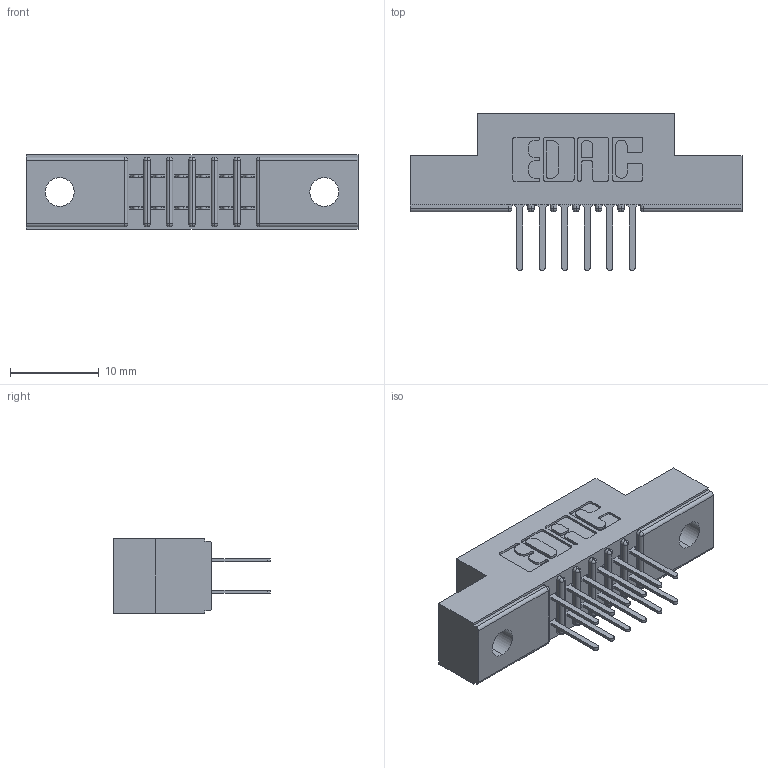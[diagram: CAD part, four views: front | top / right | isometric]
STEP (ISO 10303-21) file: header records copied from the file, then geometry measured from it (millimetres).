
FILE_DESCRIPTION (( 'STEP AP203' ), '1' );
FILE_NAME ('391-012-521-202.STEP', '2018-08-08T16:28:00', ( '' ), ( '' ), 'SwSTEP 2.0', 'SolidWorks 2016', '' );
FILE_SCHEMA (( 'CONFIG_CONTROL_DESIGN' ));
Length unit declared in the file: inch
Products named in the file (3): 341 Part_.128 (3.25) Dia Mounting Holes; 341-292-001_341-292-121; 391-012-521-202
Assembly tree (13 placements, depth 2):
  391-012-521-202
    341 Part_.128 (3.25) Dia Mounting Holes
    341-292-001_341-292-121  x12
Bounding box: 37.47 x 17.7 x 8.38 mm (x, y, z)
Volume: 2145.5 mm3; surface area: 3295.2 mm2
Topology: 13 solids, 13 shells, 908 faces, 2614 edges, 1694 vertices
Faces by surface type: plane 548, cylinder 336, sphere 14, torus 10
Entity records: 12059 total; most frequent: CARTESIAN_POINT 2006, ORIENTED_EDGE 1988, DIRECTION 1972, EDGE_CURVE 994, LINE 764, VECTOR 764, VERTEX_POINT 638, AXIS2_PLACEMENT_3D 604
